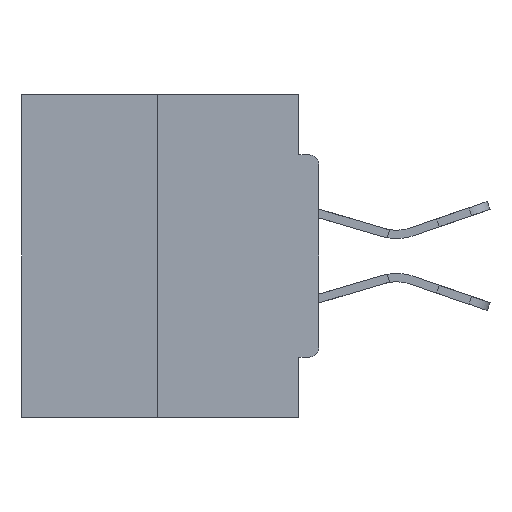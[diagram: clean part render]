
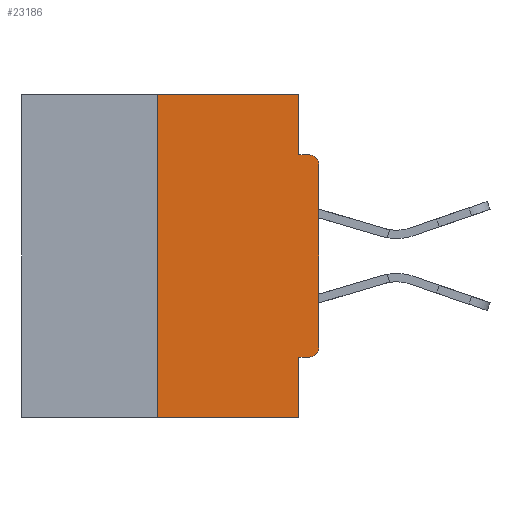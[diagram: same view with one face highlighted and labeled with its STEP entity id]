
A CAD part, left-side view. The second image highlights one B-rep face of the part: STEP entity #23186.
In plain terms, the highlighted planar face has unit normal (-1, 0, 0).
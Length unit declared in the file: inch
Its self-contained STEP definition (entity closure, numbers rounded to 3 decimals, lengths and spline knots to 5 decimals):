
#578 = LINE ( 'NONE', #27551, #5405 ) ;
#601 = EDGE_CURVE ( 'NONE', #30269, #18943, #10465, .T. ) ;
#1213 = ORIENTED_EDGE ( 'NONE', *, *, #11881, .T. ) ;
#1356 = CARTESIAN_POINT ( 'NONE',  ( 0., 0.031, -0.4065 ) ) ;
#1469 = CIRCLE ( 'NONE', #37857, 0.015 ) ;
#2365 = DIRECTION ( 'NONE',  ( 0., -1., 0. ) ) ;
#2410 = CARTESIAN_POINT ( 'NONE',  ( 0., 0.031, 0. ) ) ;
#2890 = VECTOR ( 'NONE', #11566, 39.37008 ) ;
#2957 = VERTEX_POINT ( 'NONE', #12753 ) ;
#3414 = VERTEX_POINT ( 'NONE', #13109 ) ;
#5329 = ORIENTED_EDGE ( 'NONE', *, *, #30988, .F. ) ;
#5405 = VECTOR ( 'NONE', #21589, 39.37008 ) ;
#6579 = CARTESIAN_POINT ( 'NONE',  ( 0., 0.015, -0.0935 ) ) ;
#6667 = DIRECTION ( 'NONE',  ( -1., 0., 0. ) ) ;
#6891 = ORIENTED_EDGE ( 'NONE', *, *, #21065, .T. ) ;
#8425 = FACE_OUTER_BOUND ( 'NONE', #8908, .T. ) ;
#8705 = EDGE_CURVE ( 'NONE', #39349, #27127, #578, .T. ) ;
#8830 = DIRECTION ( 'NONE',  ( 0., 0., -1. ) ) ;
#8908 = EDGE_LOOP ( 'NONE', ( #32305, #35380, #23940, #5329, #11512, #6891, #9733, #1213, #40758, #13949 ) ) ;
#9260 = LINE ( 'NONE', #27611, #2890 ) ;
#9733 = ORIENTED_EDGE ( 'NONE', *, *, #8705, .T. ) ;
#10411 = DIRECTION ( 'NONE',  ( 0., -1., 0. ) ) ;
#10465 = LINE ( 'NONE', #36215, #29619 ) ;
#11512 = ORIENTED_EDGE ( 'NONE', *, *, #38559, .F. ) ;
#11566 = DIRECTION ( 'NONE',  ( 0., -1., 0. ) ) ;
#11881 = EDGE_CURVE ( 'NONE', #27127, #36425, #1469, .T. ) ;
#12753 = CARTESIAN_POINT ( 'NONE',  ( 0., 0.25, 0. ) ) ;
#12767 = LINE ( 'NONE', #37502, #33339 ) ;
#13109 = CARTESIAN_POINT ( 'NONE',  ( 0., 0.031, -0.5 ) ) ;
#13192 = EDGE_CURVE ( 'NONE', #32993, #3414, #9260, .T. ) ;
#13677 = EDGE_CURVE ( 'NONE', #18943, #36425, #18794, .T. ) ;
#13949 = ORIENTED_EDGE ( 'NONE', *, *, #601, .F. ) ;
#15381 = DIRECTION ( 'NONE',  ( 1., 0., 0. ) ) ;
#15819 = CIRCLE ( 'NONE', #38077, 0.015 ) ;
#16594 = LINE ( 'NONE', #30076, #30524 ) ;
#17942 = AXIS2_PLACEMENT_3D ( 'NONE', #22099, #15381, #8830 ) ;
#18141 = CARTESIAN_POINT ( 'NONE',  ( 0., 0.25, -0.5 ) ) ;
#18312 = PLANE ( 'NONE',  #17942 ) ;
#18794 = LINE ( 'NONE', #21724, #34599 ) ;
#18943 = VERTEX_POINT ( 'NONE', #40956 ) ;
#19195 = DIRECTION ( 'NONE',  ( 0., 0., -1. ) ) ;
#19362 = EDGE_CURVE ( 'NONE', #32993, #2957, #12767, .T. ) ;
#19893 = LINE ( 'NONE', #35537, #34874 ) ;
#20007 = CARTESIAN_POINT ( 'NONE',  ( 0., 0., -0.1085 ) ) ;
#20751 = CARTESIAN_POINT ( 'NONE',  ( 0., 0.015, -0.4065 ) ) ;
#20813 = VERTEX_POINT ( 'NONE', #20751 ) ;
#21065 = EDGE_CURVE ( 'NONE', #20813, #39349, #15819, .T. ) ;
#21589 = DIRECTION ( 'NONE',  ( 0., 0., 1. ) ) ;
#21724 = CARTESIAN_POINT ( 'NONE',  ( 0., 0., -0.0935 ) ) ;
#22099 = CARTESIAN_POINT ( 'NONE',  ( 0., 0.46, 0. ) ) ;
#23186 = ADVANCED_FACE ( 'NONE', ( #8425 ), #18312, .F. ) ;
#23306 = DIRECTION ( 'NONE',  ( 0., 0., -1. ) ) ;
#23756 = EDGE_CURVE ( 'NONE', #2957, #30269, #19893, .T. ) ;
#23940 = ORIENTED_EDGE ( 'NONE', *, *, #13192, .T. ) ;
#24787 = DIRECTION ( 'NONE',  ( 0., 0., 1. ) ) ;
#24936 = DIRECTION ( 'NONE',  ( 0., 0., -1. ) ) ;
#25582 = CARTESIAN_POINT ( 'NONE',  ( 0., 0.015, -0.3915 ) ) ;
#27127 = VERTEX_POINT ( 'NONE', #20007 ) ;
#27551 = CARTESIAN_POINT ( 'NONE',  ( 0., 0., 0. ) ) ;
#27611 = CARTESIAN_POINT ( 'NONE',  ( 0., 0.46, -0.5 ) ) ;
#28783 = VECTOR ( 'NONE', #19195, 39.37008 ) ;
#28886 = CARTESIAN_POINT ( 'NONE',  ( 0., 0., -0.3915 ) ) ;
#28959 = VERTEX_POINT ( 'NONE', #1356 ) ;
#29619 = VECTOR ( 'NONE', #23306, 39.37008 ) ;
#30076 = CARTESIAN_POINT ( 'NONE',  ( 0., 0., -0.4065 ) ) ;
#30269 = VERTEX_POINT ( 'NONE', #2410 ) ;
#30524 = VECTOR ( 'NONE', #39599, 39.37008 ) ;
#30988 = EDGE_CURVE ( 'NONE', #28959, #3414, #35460, .T. ) ;
#32305 = ORIENTED_EDGE ( 'NONE', *, *, #23756, .F. ) ;
#32993 = VERTEX_POINT ( 'NONE', #18141 ) ;
#33339 = VECTOR ( 'NONE', #24787, 39.37008 ) ;
#34599 = VECTOR ( 'NONE', #2365, 39.37008 ) ;
#34874 = VECTOR ( 'NONE', #10411, 39.37008 ) ;
#35380 = ORIENTED_EDGE ( 'NONE', *, *, #19362, .F. ) ;
#35460 = LINE ( 'NONE', #38629, #28783 ) ;
#35537 = CARTESIAN_POINT ( 'NONE',  ( 0., 0.46, 0. ) ) ;
#35574 = CARTESIAN_POINT ( 'NONE',  ( 0., 0.015, -0.1085 ) ) ;
#36215 = CARTESIAN_POINT ( 'NONE',  ( 0., 0.031, 0. ) ) ;
#36425 = VERTEX_POINT ( 'NONE', #6579 ) ;
#37502 = CARTESIAN_POINT ( 'NONE',  ( 0., 0.25, 0. ) ) ;
#37857 = AXIS2_PLACEMENT_3D ( 'NONE', #35574, #6667, #38748 ) ;
#38077 = AXIS2_PLACEMENT_3D ( 'NONE', #25582, #38476, #24936 ) ;
#38476 = DIRECTION ( 'NONE',  ( -1., 0., 0. ) ) ;
#38559 = EDGE_CURVE ( 'NONE', #20813, #28959, #16594, .T. ) ;
#38629 = CARTESIAN_POINT ( 'NONE',  ( 0., 0.031, -0.5 ) ) ;
#38748 = DIRECTION ( 'NONE',  ( 0., 0., -1. ) ) ;
#39349 = VERTEX_POINT ( 'NONE', #28886 ) ;
#39599 = DIRECTION ( 'NONE',  ( 0., 1., 0. ) ) ;
#40758 = ORIENTED_EDGE ( 'NONE', *, *, #13677, .F. ) ;
#40956 = CARTESIAN_POINT ( 'NONE',  ( 0., 0.031, -0.0935 ) ) ;
